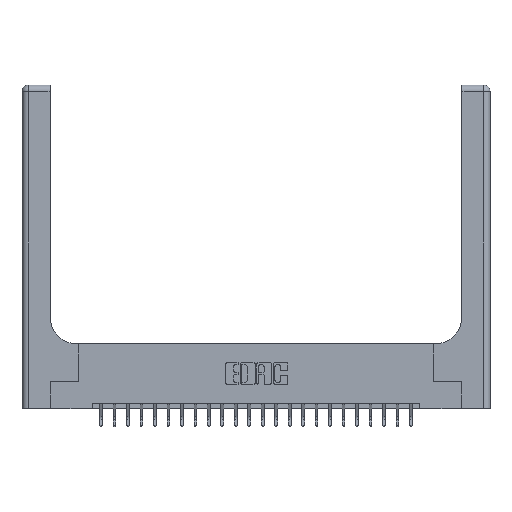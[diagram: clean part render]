
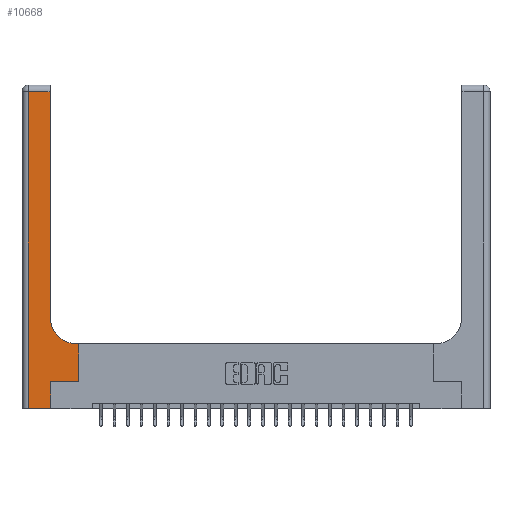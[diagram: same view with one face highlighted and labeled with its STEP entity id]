
A CAD part, top view. The second image highlights one B-rep face of the part: STEP entity #10668.
In plain terms, the highlighted planar face has unit normal (0, 0, 1).
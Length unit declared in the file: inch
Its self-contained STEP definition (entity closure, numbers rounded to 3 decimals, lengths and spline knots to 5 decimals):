
#17 = CARTESIAN_POINT ( 'NONE',  ( 0.528, 0.6, 0.37 ) ) ;
#25 = EDGE_CURVE ( 'NONE', #4357, #6221, #7192, .T. ) ;
#434 = ORIENTED_EDGE ( 'NONE', *, *, #3027, .T. ) ;
#1062 = VERTEX_POINT ( 'NONE', #9601 ) ;
#1129 = VERTEX_POINT ( 'NONE', #22942 ) ;
#1940 = AXIS2_PLACEMENT_3D ( 'NONE', #4907, #17511, #15942 ) ;
#2883 = LINE ( 'NONE', #11972, #10023 ) ;
#3027 = EDGE_CURVE ( 'NONE', #16610, #11314, #21361, .T. ) ;
#3422 = CARTESIAN_POINT ( 'NONE',  ( 0.51, 0.85, 0.37 ) ) ;
#4151 = ORIENTED_EDGE ( 'NONE', *, *, #22964, .T. ) ;
#4357 = VERTEX_POINT ( 'NONE', #19079 ) ;
#4574 = CIRCLE ( 'NONE', #8805, 0.25 ) ;
#4907 = CARTESIAN_POINT ( 'NONE',  ( 0., 3., 0.37 ) ) ;
#5151 = VERTEX_POINT ( 'NONE', #22411 ) ;
#5245 = LINE ( 'NONE', #12634, #20474 ) ;
#5412 = ORIENTED_EDGE ( 'NONE', *, *, #23451, .T. ) ;
#5988 = VECTOR ( 'NONE', #22831, 39.37008 ) ;
#6080 = EDGE_CURVE ( 'NONE', #5151, #15224, #4574, .T. ) ;
#6221 = VERTEX_POINT ( 'NONE', #17223 ) ;
#6322 = LINE ( 'NONE', #15432, #5988 ) ;
#6342 = EDGE_CURVE ( 'NONE', #1129, #12515, #8475, .T. ) ;
#6389 = CARTESIAN_POINT ( 'NONE',  ( 0.265, 0.25, 0.37 ) ) ;
#6535 = ORIENTED_EDGE ( 'NONE', *, *, #6677, .T. ) ;
#6659 = DIRECTION ( 'NONE',  ( 0., 1., 0. ) ) ;
#6677 = EDGE_CURVE ( 'NONE', #11314, #1129, #2883, .T. ) ;
#6740 = DIRECTION ( 'NONE',  ( 1., 0., 0. ) ) ;
#6777 = CARTESIAN_POINT ( 'NONE',  ( 0.265, 0., 0.37 ) ) ;
#6818 = DIRECTION ( 'NONE',  ( 0., 1., 0. ) ) ;
#7192 = LINE ( 'NONE', #20180, #20022 ) ;
#7568 = ORIENTED_EDGE ( 'NONE', *, *, #9164, .T. ) ;
#7682 = EDGE_LOOP ( 'NONE', ( #5412, #4151, #18712, #7568, #434, #6535, #15689, #9220, #18485 ) ) ;
#8475 = LINE ( 'NONE', #23274, #10010 ) ;
#8805 = AXIS2_PLACEMENT_3D ( 'NONE', #3422, #10799, #23754 ) ;
#9164 = EDGE_CURVE ( 'NONE', #6221, #16610, #20087, .T. ) ;
#9220 = ORIENTED_EDGE ( 'NONE', *, *, #18368, .T. ) ;
#9601 = CARTESIAN_POINT ( 'NONE',  ( 0.26, 2.94, 0.37 ) ) ;
#9996 = PLANE ( 'NONE',  #1940 ) ;
#10010 = VECTOR ( 'NONE', #6659, 39.37008 ) ;
#10023 = VECTOR ( 'NONE', #6740, 39.37008 ) ;
#10668 = ADVANCED_FACE ( 'NONE', ( #17631 ), #9996, .F. ) ;
#10718 = LINE ( 'NONE', #23795, #23538 ) ;
#10799 = DIRECTION ( 'NONE',  ( 0., 0., -1. ) ) ;
#10861 = CARTESIAN_POINT ( 'NONE',  ( 0., 0., 0.37 ) ) ;
#11314 = VERTEX_POINT ( 'NONE', #6389 ) ;
#11972 = CARTESIAN_POINT ( 'NONE',  ( 0.265, 0.25, 0.37 ) ) ;
#12515 = VERTEX_POINT ( 'NONE', #17 ) ;
#12634 = CARTESIAN_POINT ( 'NONE',  ( 0.26, 3., 0.37 ) ) ;
#13492 = VECTOR ( 'NONE', #18373, 39.37008 ) ;
#14362 = CARTESIAN_POINT ( 'NONE',  ( 0.265, 0., 0.37 ) ) ;
#14481 = VECTOR ( 'NONE', #19652, 39.37008 ) ;
#15224 = VERTEX_POINT ( 'NONE', #23102 ) ;
#15432 = CARTESIAN_POINT ( 'NONE',  ( 0.26, 0.6, 0.37 ) ) ;
#15689 = ORIENTED_EDGE ( 'NONE', *, *, #6342, .T. ) ;
#15942 = DIRECTION ( 'NONE',  ( -1., 0., 0. ) ) ;
#16610 = VERTEX_POINT ( 'NONE', #14362 ) ;
#17223 = CARTESIAN_POINT ( 'NONE',  ( 0.06, 0., 0.37 ) ) ;
#17511 = DIRECTION ( 'NONE',  ( 0., 0., -1. ) ) ;
#17631 = FACE_OUTER_BOUND ( 'NONE', #7682, .T. ) ;
#18126 = DIRECTION ( 'NONE',  ( -1., 0., 0. ) ) ;
#18368 = EDGE_CURVE ( 'NONE', #12515, #5151, #6322, .T. ) ;
#18373 = DIRECTION ( 'NONE',  ( 1., 0., 0. ) ) ;
#18485 = ORIENTED_EDGE ( 'NONE', *, *, #6080, .T. ) ;
#18712 = ORIENTED_EDGE ( 'NONE', *, *, #25, .T. ) ;
#19079 = CARTESIAN_POINT ( 'NONE',  ( 0.06, 2.94, 0.37 ) ) ;
#19652 = DIRECTION ( 'NONE',  ( 0., 1., 0. ) ) ;
#20022 = VECTOR ( 'NONE', #20408, 39.37008 ) ;
#20087 = LINE ( 'NONE', #10861, #13492 ) ;
#20180 = CARTESIAN_POINT ( 'NONE',  ( 0.06, 3., 0.37 ) ) ;
#20408 = DIRECTION ( 'NONE',  ( 0., -1., 0. ) ) ;
#20474 = VECTOR ( 'NONE', #6818, 39.37008 ) ;
#21361 = LINE ( 'NONE', #6777, #14481 ) ;
#22411 = CARTESIAN_POINT ( 'NONE',  ( 0.51, 0.6, 0.37 ) ) ;
#22831 = DIRECTION ( 'NONE',  ( -1., 0., 0. ) ) ;
#22942 = CARTESIAN_POINT ( 'NONE',  ( 0.528, 0.25, 0.37 ) ) ;
#22964 = EDGE_CURVE ( 'NONE', #1062, #4357, #10718, .T. ) ;
#23102 = CARTESIAN_POINT ( 'NONE',  ( 0.26, 0.85, 0.37 ) ) ;
#23274 = CARTESIAN_POINT ( 'NONE',  ( 0.528, 0.25, 0.37 ) ) ;
#23451 = EDGE_CURVE ( 'NONE', #15224, #1062, #5245, .T. ) ;
#23538 = VECTOR ( 'NONE', #18126, 39.37008 ) ;
#23754 = DIRECTION ( 'NONE',  ( 1., 0., 0. ) ) ;
#23795 = CARTESIAN_POINT ( 'NONE',  ( 0., 2.94, 0.37 ) ) ;
